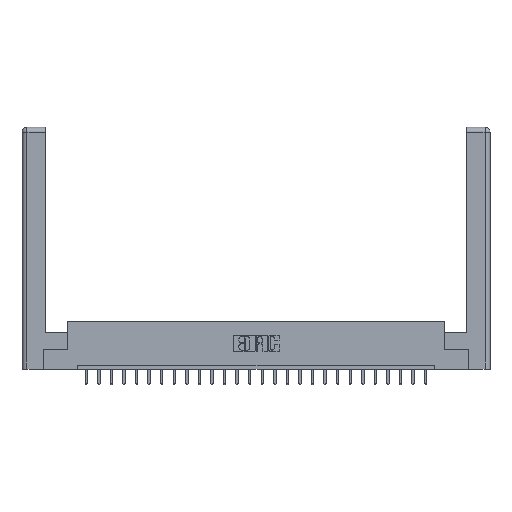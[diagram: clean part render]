
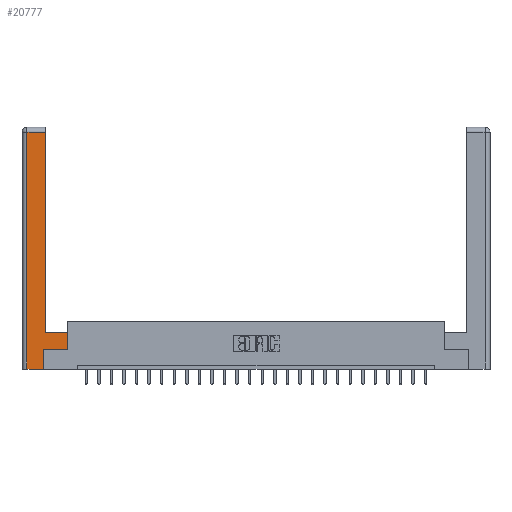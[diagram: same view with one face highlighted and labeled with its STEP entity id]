
A CAD part, top view. The second image highlights one B-rep face of the part: STEP entity #20777.
In plain terms, the highlighted planar face has unit normal (0, 0, 1).
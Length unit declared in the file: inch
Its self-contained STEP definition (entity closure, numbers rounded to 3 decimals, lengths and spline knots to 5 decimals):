
#1260 = CARTESIAN_POINT ( 'NONE',  ( 0.0615, 0., 0. ) ) ;
#1349 = VECTOR ( 'NONE', #20520, 39.37008 ) ;
#2198 = EDGE_LOOP ( 'NONE', ( #6890, #11720, #6668, #4907, #5766, #17722, #14575, #12679 ) ) ;
#2914 = CARTESIAN_POINT ( 'NONE',  ( 0.265, 0.245, 0. ) ) ;
#2990 = CARTESIAN_POINT ( 'NONE',  ( 0., 0., 0. ) ) ;
#4664 = DIRECTION ( 'NONE',  ( 0., 1., 0. ) ) ;
#4907 = ORIENTED_EDGE ( 'NONE', *, *, #6168, .T. ) ;
#5573 = CARTESIAN_POINT ( 'NONE',  ( 0.265, 0., 0. ) ) ;
#5749 = CARTESIAN_POINT ( 'NONE',  ( 0.0615, 2.94, 0. ) ) ;
#5766 = ORIENTED_EDGE ( 'NONE', *, *, #14165, .T. ) ;
#5974 = CARTESIAN_POINT ( 'NONE',  ( 0.0615, 2.94, 0. ) ) ;
#6168 = EDGE_CURVE ( 'NONE', #24165, #11469, #16077, .T. ) ;
#6189 = CARTESIAN_POINT ( 'NONE',  ( 0.295, 0.45, 0. ) ) ;
#6259 = EDGE_CURVE ( 'NONE', #18550, #22825, #21309, .T. ) ;
#6567 = LINE ( 'NONE', #12737, #1349 ) ;
#6668 = ORIENTED_EDGE ( 'NONE', *, *, #12005, .T. ) ;
#6890 = ORIENTED_EDGE ( 'NONE', *, *, #24809, .T. ) ;
#7163 = VECTOR ( 'NONE', #11189, 39.37008 ) ;
#7541 = DIRECTION ( 'NONE',  ( -1., 0., 0. ) ) ;
#7644 = CARTESIAN_POINT ( 'NONE',  ( 0.565, 0.45, 0. ) ) ;
#7818 = LINE ( 'NONE', #6189, #24957 ) ;
#9610 = LINE ( 'NONE', #16212, #20927 ) ;
#10163 = DIRECTION ( 'NONE',  ( -1., 0., 0. ) ) ;
#10237 = AXIS2_PLACEMENT_3D ( 'NONE', #2990, #24391, #24288 ) ;
#10284 = VERTEX_POINT ( 'NONE', #25051 ) ;
#10970 = VERTEX_POINT ( 'NONE', #24984 ) ;
#11189 = DIRECTION ( 'NONE',  ( 0., 1., 0. ) ) ;
#11304 = CARTESIAN_POINT ( 'NONE',  ( 0.565, 0.45, 0. ) ) ;
#11469 = VERTEX_POINT ( 'NONE', #16947 ) ;
#11720 = ORIENTED_EDGE ( 'NONE', *, *, #18811, .T. ) ;
#12005 = EDGE_CURVE ( 'NONE', #13550, #24165, #21090, .T. ) ;
#12679 = ORIENTED_EDGE ( 'NONE', *, *, #12832, .T. ) ;
#12737 = CARTESIAN_POINT ( 'NONE',  ( 0.265, 0.245, 0. ) ) ;
#12832 = EDGE_CURVE ( 'NONE', #12955, #10970, #7818, .T. ) ;
#12955 = VERTEX_POINT ( 'NONE', #11304 ) ;
#13550 = VERTEX_POINT ( 'NONE', #5974 ) ;
#13580 = DIRECTION ( 'NONE',  ( 1., 0., 0. ) ) ;
#14165 = EDGE_CURVE ( 'NONE', #11469, #18550, #6567, .T. ) ;
#14575 = ORIENTED_EDGE ( 'NONE', *, *, #18828, .T. ) ;
#15008 = DIRECTION ( 'NONE',  ( 0., -1., 0. ) ) ;
#15171 = CARTESIAN_POINT ( 'NONE',  ( 0.565, 0.245, 0. ) ) ;
#16077 = LINE ( 'NONE', #5573, #18826 ) ;
#16212 = CARTESIAN_POINT ( 'NONE',  ( 0.295, 3., 0. ) ) ;
#16947 = CARTESIAN_POINT ( 'NONE',  ( 0.265, 0., 0. ) ) ;
#17548 = VECTOR ( 'NONE', #7541, 39.37008 ) ;
#17722 = ORIENTED_EDGE ( 'NONE', *, *, #6259, .T. ) ;
#18550 = VERTEX_POINT ( 'NONE', #2914 ) ;
#18762 = LINE ( 'NONE', #7644, #7163 ) ;
#18811 = EDGE_CURVE ( 'NONE', #10284, #13550, #22816, .T. ) ;
#18826 = VECTOR ( 'NONE', #19411, 39.37008 ) ;
#18828 = EDGE_CURVE ( 'NONE', #22825, #12955, #18762, .T. ) ;
#19153 = CARTESIAN_POINT ( 'NONE',  ( 0.0615, 0., 0. ) ) ;
#19411 = DIRECTION ( 'NONE',  ( 1., 0., 0. ) ) ;
#20061 = VECTOR ( 'NONE', #13580, 39.37008 ) ;
#20334 = PLANE ( 'NONE',  #10237 ) ;
#20461 = VECTOR ( 'NONE', #15008, 39.37008 ) ;
#20520 = DIRECTION ( 'NONE',  ( 0., 1., 0. ) ) ;
#20526 = FACE_OUTER_BOUND ( 'NONE', #2198, .T. ) ;
#20777 = ADVANCED_FACE ( 'NONE', ( #20526 ), #20334, .F. ) ;
#20927 = VECTOR ( 'NONE', #4664, 39.37008 ) ;
#21090 = LINE ( 'NONE', #1260, #20461 ) ;
#21309 = LINE ( 'NONE', #25351, #20061 ) ;
#22816 = LINE ( 'NONE', #5749, #17548 ) ;
#22825 = VERTEX_POINT ( 'NONE', #15171 ) ;
#24165 = VERTEX_POINT ( 'NONE', #19153 ) ;
#24288 = DIRECTION ( 'NONE',  ( -1., 0., 0. ) ) ;
#24391 = DIRECTION ( 'NONE',  ( 0., 0., -1. ) ) ;
#24809 = EDGE_CURVE ( 'NONE', #10970, #10284, #9610, .T. ) ;
#24957 = VECTOR ( 'NONE', #10163, 39.37008 ) ;
#24984 = CARTESIAN_POINT ( 'NONE',  ( 0.295, 0.45, 0. ) ) ;
#25051 = CARTESIAN_POINT ( 'NONE',  ( 0.295, 2.94, 0. ) ) ;
#25351 = CARTESIAN_POINT ( 'NONE',  ( 0.565, 0.245, 0. ) ) ;
